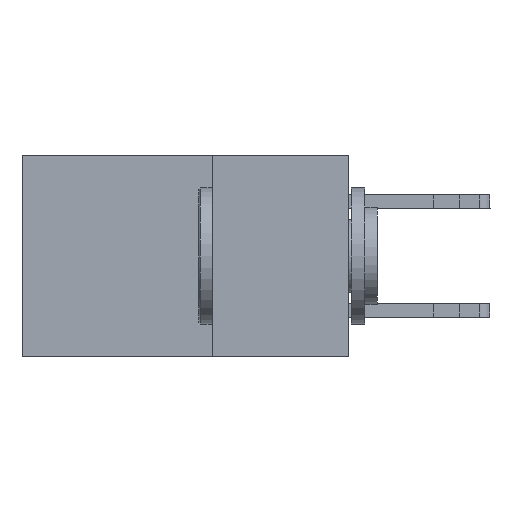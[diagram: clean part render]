
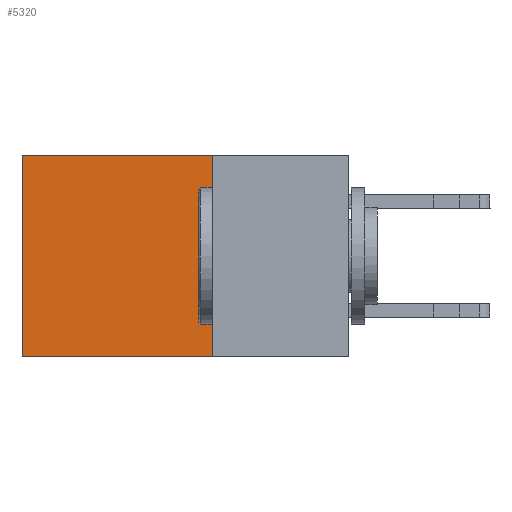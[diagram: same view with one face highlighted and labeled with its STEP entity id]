
A CAD part, left-side view. The second image highlights one B-rep face of the part: STEP entity #5320.
In plain terms, the highlighted planar face has unit normal (-1, 0, 0).
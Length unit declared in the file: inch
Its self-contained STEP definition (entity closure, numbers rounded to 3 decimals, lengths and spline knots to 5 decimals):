
#596 = VECTOR ( 'NONE', #18037, 39.37008 ) ;
#763 = EDGE_CURVE ( 'NONE', #4623, #7897, #19353, .T. ) ;
#1189 = LINE ( 'NONE', #4119, #596 ) ;
#1396 = AXIS2_PLACEMENT_3D ( 'NONE', #18303, #9029, #10733 ) ;
#1635 = VERTEX_POINT ( 'NONE', #15010 ) ;
#2782 = EDGE_CURVE ( 'NONE', #4623, #1635, #17267, .T. ) ;
#2792 = CARTESIAN_POINT ( 'NONE',  ( 0.2615, 0.25, 0. ) ) ;
#3518 = ORIENTED_EDGE ( 'NONE', *, *, #18823, .F. ) ;
#4119 = CARTESIAN_POINT ( 'NONE',  ( 0.2615, 0.25, -0.37 ) ) ;
#4312 = CARTESIAN_POINT ( 'NONE',  ( 0.2615, 0.6, -0.37 ) ) ;
#4623 = VERTEX_POINT ( 'NONE', #9592 ) ;
#4889 = FACE_OUTER_BOUND ( 'NONE', #7615, .T. ) ;
#5320 = ADVANCED_FACE ( 'NONE', ( #4889 ), #6401, .F. ) ;
#5417 = VECTOR ( 'NONE', #12182, 39.37008 ) ;
#6401 = PLANE ( 'NONE',  #1396 ) ;
#6798 = CARTESIAN_POINT ( 'NONE',  ( 0.2615, 0.25, -0.37 ) ) ;
#7427 = VECTOR ( 'NONE', #8951, 39.37008 ) ;
#7469 = CARTESIAN_POINT ( 'NONE',  ( 0.2615, 0.6, -0.37 ) ) ;
#7615 = EDGE_LOOP ( 'NONE', ( #14038, #3518, #9967, #8126 ) ) ;
#7897 = VERTEX_POINT ( 'NONE', #12032 ) ;
#8104 = DIRECTION ( 'NONE',  ( 0., 0., -1. ) ) ;
#8126 = ORIENTED_EDGE ( 'NONE', *, *, #763, .T. ) ;
#8827 = EDGE_CURVE ( 'NONE', #7897, #10202, #16324, .T. ) ;
#8951 = DIRECTION ( 'NONE',  ( 0., 1., 0. ) ) ;
#9029 = DIRECTION ( 'NONE',  ( 1., 0., 0. ) ) ;
#9592 = CARTESIAN_POINT ( 'NONE',  ( 0.2615, 0.25, 0. ) ) ;
#9967 = ORIENTED_EDGE ( 'NONE', *, *, #2782, .F. ) ;
#10202 = VERTEX_POINT ( 'NONE', #7469 ) ;
#10733 = DIRECTION ( 'NONE',  ( 0., 0., -1. ) ) ;
#12032 = CARTESIAN_POINT ( 'NONE',  ( 0.2615, 0.6, 0. ) ) ;
#12182 = DIRECTION ( 'NONE',  ( 0., 0., -1. ) ) ;
#13542 = VECTOR ( 'NONE', #8104, 39.37008 ) ;
#14038 = ORIENTED_EDGE ( 'NONE', *, *, #8827, .T. ) ;
#15010 = CARTESIAN_POINT ( 'NONE',  ( 0.2615, 0.25, -0.37 ) ) ;
#16324 = LINE ( 'NONE', #4312, #5417 ) ;
#17267 = LINE ( 'NONE', #6798, #13542 ) ;
#18037 = DIRECTION ( 'NONE',  ( 0., 1., 0. ) ) ;
#18303 = CARTESIAN_POINT ( 'NONE',  ( 0.2615, 0.25, -0.37 ) ) ;
#18823 = EDGE_CURVE ( 'NONE', #1635, #10202, #1189, .T. ) ;
#19353 = LINE ( 'NONE', #2792, #7427 ) ;
